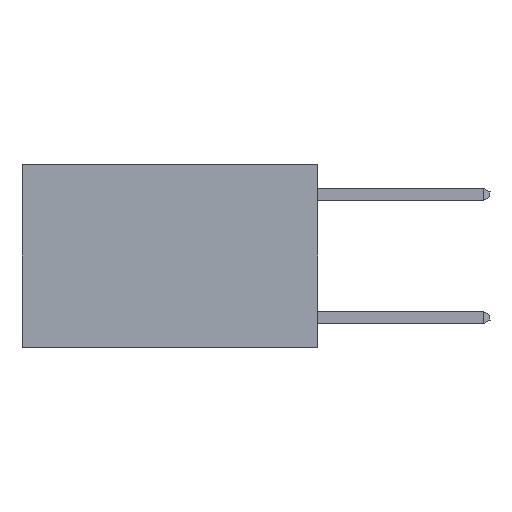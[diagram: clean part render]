
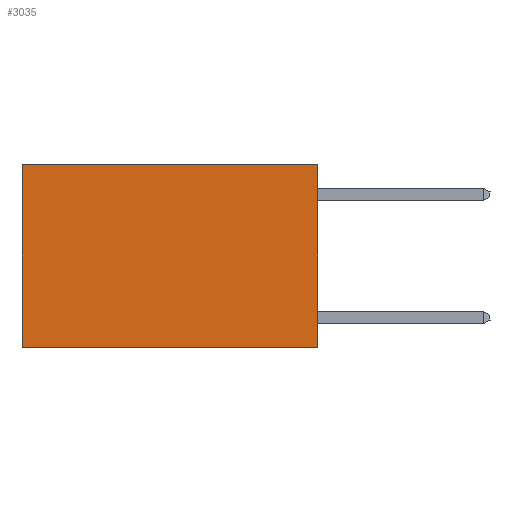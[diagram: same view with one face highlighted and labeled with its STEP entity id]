
A CAD part, left-side view. The second image highlights one B-rep face of the part: STEP entity #3035.
In plain terms, the highlighted planar face has unit normal (-1, 0, 0).
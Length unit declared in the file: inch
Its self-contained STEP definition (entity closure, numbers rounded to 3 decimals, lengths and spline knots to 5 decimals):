
#123 = DIRECTION ( 'NONE',  ( 0., 0., -1. ) ) ;
#125 = ORIENTED_EDGE ( 'NONE', *, *, #13695, .T. ) ;
#1831 = VERTEX_POINT ( 'NONE', #17644 ) ;
#2186 = FACE_OUTER_BOUND ( 'NONE', #4666, .T. ) ;
#2353 = VECTOR ( 'NONE', #123, 39.37008 ) ;
#2647 = ORIENTED_EDGE ( 'NONE', *, *, #15434, .F. ) ;
#3035 = ADVANCED_FACE ( 'NONE', ( #2186 ), #12408, .F. ) ;
#3202 = DIRECTION ( 'NONE',  ( 0., 1., 0. ) ) ;
#4316 = EDGE_CURVE ( 'NONE', #1831, #15064, #7382, .T. ) ;
#4666 = EDGE_LOOP ( 'NONE', ( #125, #2647, #18103, #10787 ) ) ;
#5533 = VECTOR ( 'NONE', #8705, 39.37008 ) ;
#5846 = CARTESIAN_POINT ( 'NONE',  ( 0.2625, 0.6, 0. ) ) ;
#7131 = CARTESIAN_POINT ( 'NONE',  ( 0.2625, 0., -0.37 ) ) ;
#7382 = LINE ( 'NONE', #15141, #2353 ) ;
#8589 = LINE ( 'NONE', #9244, #12475 ) ;
#8705 = DIRECTION ( 'NONE',  ( 0., 0., -1. ) ) ;
#9244 = CARTESIAN_POINT ( 'NONE',  ( 0.2625, 0., 0. ) ) ;
#10787 = ORIENTED_EDGE ( 'NONE', *, *, #14227, .T. ) ;
#10984 = CARTESIAN_POINT ( 'NONE',  ( 0.2625, 0.6, -0.37 ) ) ;
#11981 = CARTESIAN_POINT ( 'NONE',  ( 0.2625, 0.6, 0. ) ) ;
#12314 = DIRECTION ( 'NONE',  ( 1., 0., 0. ) ) ;
#12408 = PLANE ( 'NONE',  #15624 ) ;
#12475 = VECTOR ( 'NONE', #16698, 39.37008 ) ;
#12515 = VERTEX_POINT ( 'NONE', #10984 ) ;
#13695 = EDGE_CURVE ( 'NONE', #17711, #12515, #17925, .T. ) ;
#14227 = EDGE_CURVE ( 'NONE', #1831, #17711, #8589, .T. ) ;
#15064 = VERTEX_POINT ( 'NONE', #7131 ) ;
#15141 = CARTESIAN_POINT ( 'NONE',  ( 0.2625, 0., 0. ) ) ;
#15434 = EDGE_CURVE ( 'NONE', #15064, #12515, #18413, .T. ) ;
#15598 = VECTOR ( 'NONE', #3202, 39.37008 ) ;
#15624 = AXIS2_PLACEMENT_3D ( 'NONE', #18583, #12314, #18376 ) ;
#16698 = DIRECTION ( 'NONE',  ( 0., 1., 0. ) ) ;
#16743 = CARTESIAN_POINT ( 'NONE',  ( 0.2625, 0., -0.37 ) ) ;
#17644 = CARTESIAN_POINT ( 'NONE',  ( 0.2625, 0., 0. ) ) ;
#17711 = VERTEX_POINT ( 'NONE', #11981 ) ;
#17925 = LINE ( 'NONE', #5846, #5533 ) ;
#18103 = ORIENTED_EDGE ( 'NONE', *, *, #4316, .F. ) ;
#18376 = DIRECTION ( 'NONE',  ( 0., 0., -1. ) ) ;
#18413 = LINE ( 'NONE', #16743, #15598 ) ;
#18583 = CARTESIAN_POINT ( 'NONE',  ( 0.2625, 0., 0. ) ) ;
